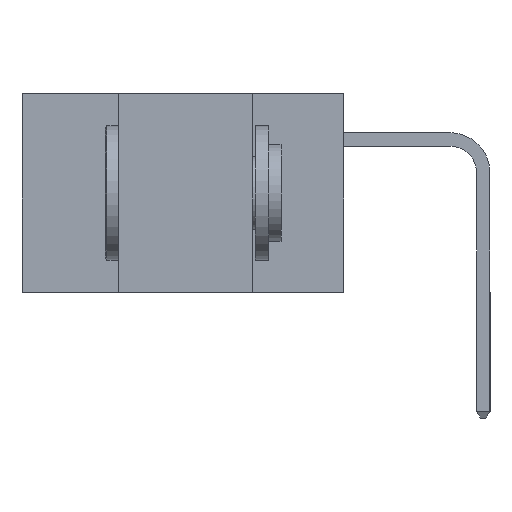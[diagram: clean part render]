
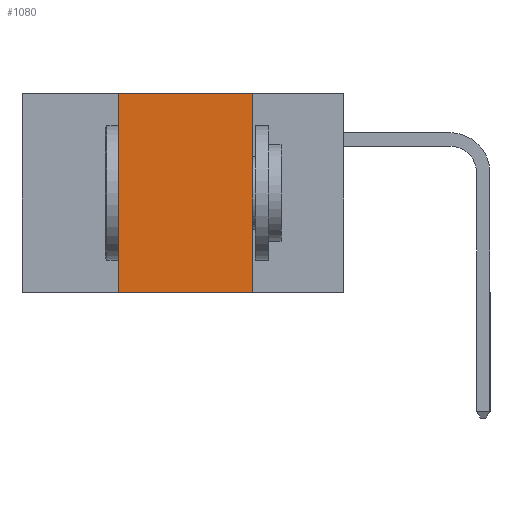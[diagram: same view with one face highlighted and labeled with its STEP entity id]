
A CAD part, left-side view. The second image highlights one B-rep face of the part: STEP entity #1080.
In plain terms, the highlighted planar face has unit normal (-1, 0, 0).
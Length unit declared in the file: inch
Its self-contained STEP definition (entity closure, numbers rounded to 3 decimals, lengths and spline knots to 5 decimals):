
#1080 = ADVANCED_FACE ( 'NONE', ( #21437 ), #27036, .F. ) ;
#2644 = LINE ( 'NONE', #17914, #22235 ) ;
#3362 = VECTOR ( 'NONE', #26761, 39.37008 ) ;
#7647 = EDGE_LOOP ( 'NONE', ( #28049, #7975, #11270, #9980 ) ) ;
#7975 = ORIENTED_EDGE ( 'NONE', *, *, #21905, .F. ) ;
#8050 = DIRECTION ( 'NONE',  ( 0., 0., 1. ) ) ;
#8750 = EDGE_CURVE ( 'NONE', #21404, #11844, #2644, .T. ) ;
#9826 = VERTEX_POINT ( 'NONE', #19065 ) ;
#9980 = ORIENTED_EDGE ( 'NONE', *, *, #15910, .T. ) ;
#11033 = CARTESIAN_POINT ( 'NONE',  ( 0., 0.6, -0.37 ) ) ;
#11270 = ORIENTED_EDGE ( 'NONE', *, *, #8750, .F. ) ;
#11760 = CARTESIAN_POINT ( 'NONE',  ( 0., 0.42, 0. ) ) ;
#11844 = VERTEX_POINT ( 'NONE', #11760 ) ;
#14736 = CARTESIAN_POINT ( 'NONE',  ( 0., 0.17, 0. ) ) ;
#15910 = EDGE_CURVE ( 'NONE', #21404, #19383, #31234, .T. ) ;
#15996 = AXIS2_PLACEMENT_3D ( 'NONE', #21870, #28687, #28330 ) ;
#16244 = CARTESIAN_POINT ( 'NONE',  ( 0., 0.17, -0.37 ) ) ;
#16300 = DIRECTION ( 'NONE',  ( 0., -1., 0. ) ) ;
#17914 = CARTESIAN_POINT ( 'NONE',  ( 0., 0.42, 0. ) ) ;
#19065 = CARTESIAN_POINT ( 'NONE',  ( 0., 0.17, 0. ) ) ;
#19383 = VERTEX_POINT ( 'NONE', #16244 ) ;
#21011 = VECTOR ( 'NONE', #16300, 39.37008 ) ;
#21404 = VERTEX_POINT ( 'NONE', #28347 ) ;
#21437 = FACE_OUTER_BOUND ( 'NONE', #7647, .T. ) ;
#21769 = LINE ( 'NONE', #23508, #21011 ) ;
#21870 = CARTESIAN_POINT ( 'NONE',  ( 0., 0.6, 0. ) ) ;
#21905 = EDGE_CURVE ( 'NONE', #11844, #9826, #21769, .T. ) ;
#22235 = VECTOR ( 'NONE', #8050, 39.37008 ) ;
#23508 = CARTESIAN_POINT ( 'NONE',  ( 0., 0.6, 0. ) ) ;
#23671 = LINE ( 'NONE', #14736, #3362 ) ;
#24969 = VECTOR ( 'NONE', #27994, 39.37008 ) ;
#26761 = DIRECTION ( 'NONE',  ( 0., 0., -1. ) ) ;
#27036 = PLANE ( 'NONE',  #15996 ) ;
#27994 = DIRECTION ( 'NONE',  ( 0., -1., 0. ) ) ;
#28049 = ORIENTED_EDGE ( 'NONE', *, *, #29583, .F. ) ;
#28330 = DIRECTION ( 'NONE',  ( 0., 0., -1. ) ) ;
#28347 = CARTESIAN_POINT ( 'NONE',  ( 0., 0.42, -0.37 ) ) ;
#28687 = DIRECTION ( 'NONE',  ( 1., 0., 0. ) ) ;
#29583 = EDGE_CURVE ( 'NONE', #9826, #19383, #23671, .T. ) ;
#31234 = LINE ( 'NONE', #11033, #24969 ) ;
